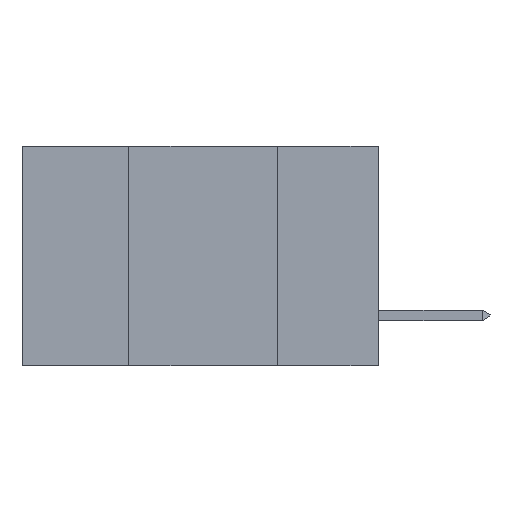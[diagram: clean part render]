
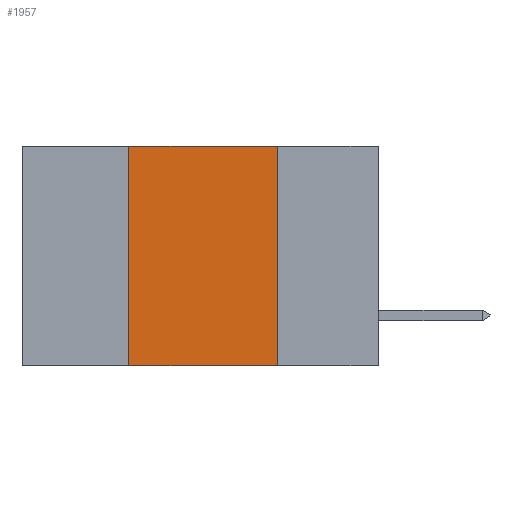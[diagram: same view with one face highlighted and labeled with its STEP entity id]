
A CAD part, left-side view. The second image highlights one B-rep face of the part: STEP entity #1957.
In plain terms, the highlighted planar face has unit normal (-1, 0, 0).
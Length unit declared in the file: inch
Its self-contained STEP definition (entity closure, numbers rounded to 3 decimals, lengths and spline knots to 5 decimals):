
#370 = ORIENTED_EDGE ( 'NONE', *, *, #18347, .T. ) ;
#516 = VECTOR ( 'NONE', #3709, 39.37008 ) ;
#571 = VECTOR ( 'NONE', #15770, 39.37008 ) ;
#1002 = VERTEX_POINT ( 'NONE', #11960 ) ;
#1957 = ADVANCED_FACE ( 'NONE', ( #3075 ), #7183, .F. ) ;
#2861 = EDGE_CURVE ( 'NONE', #17517, #3529, #12610, .T. ) ;
#3075 = FACE_OUTER_BOUND ( 'NONE', #13090, .T. ) ;
#3529 = VERTEX_POINT ( 'NONE', #19596 ) ;
#3709 = DIRECTION ( 'NONE',  ( 0., 0., -1. ) ) ;
#4154 = DIRECTION ( 'NONE',  ( 0., 0., 1. ) ) ;
#7183 = PLANE ( 'NONE',  #22172 ) ;
#7394 = EDGE_CURVE ( 'NONE', #22367, #17517, #10918, .T. ) ;
#8361 = CARTESIAN_POINT ( 'NONE',  ( 0., 0.6, -0.37 ) ) ;
#8960 = VECTOR ( 'NONE', #4154, 39.37008 ) ;
#10918 = LINE ( 'NONE', #12962, #13912 ) ;
#11226 = LINE ( 'NONE', #20807, #8960 ) ;
#11960 = CARTESIAN_POINT ( 'NONE',  ( 0., 0.42, -0.37 ) ) ;
#12610 = LINE ( 'NONE', #24008, #516 ) ;
#12819 = EDGE_CURVE ( 'NONE', #1002, #22367, #11226, .T. ) ;
#12962 = CARTESIAN_POINT ( 'NONE',  ( 0., 0.6, 0. ) ) ;
#13090 = EDGE_LOOP ( 'NONE', ( #15462, #20037, #16574, #370 ) ) ;
#13182 = CARTESIAN_POINT ( 'NONE',  ( 0., 0.17, 0. ) ) ;
#13849 = LINE ( 'NONE', #8361, #571 ) ;
#13912 = VECTOR ( 'NONE', #18550, 39.37008 ) ;
#14257 = CARTESIAN_POINT ( 'NONE',  ( 0., 0.6, 0. ) ) ;
#15462 = ORIENTED_EDGE ( 'NONE', *, *, #2861, .F. ) ;
#15770 = DIRECTION ( 'NONE',  ( 0., -1., 0. ) ) ;
#16437 = DIRECTION ( 'NONE',  ( 1., 0., 0. ) ) ;
#16574 = ORIENTED_EDGE ( 'NONE', *, *, #12819, .F. ) ;
#17517 = VERTEX_POINT ( 'NONE', #13182 ) ;
#18347 = EDGE_CURVE ( 'NONE', #1002, #3529, #13849, .T. ) ;
#18550 = DIRECTION ( 'NONE',  ( 0., -1., 0. ) ) ;
#19596 = CARTESIAN_POINT ( 'NONE',  ( 0., 0.17, -0.37 ) ) ;
#20037 = ORIENTED_EDGE ( 'NONE', *, *, #7394, .F. ) ;
#20667 = CARTESIAN_POINT ( 'NONE',  ( 0., 0.42, 0. ) ) ;
#20807 = CARTESIAN_POINT ( 'NONE',  ( 0., 0.42, -0.37 ) ) ;
#22172 = AXIS2_PLACEMENT_3D ( 'NONE', #14257, #16437, #23863 ) ;
#22367 = VERTEX_POINT ( 'NONE', #20667 ) ;
#23863 = DIRECTION ( 'NONE',  ( 0., 0., -1. ) ) ;
#24008 = CARTESIAN_POINT ( 'NONE',  ( 0., 0.17, -0.37 ) ) ;
